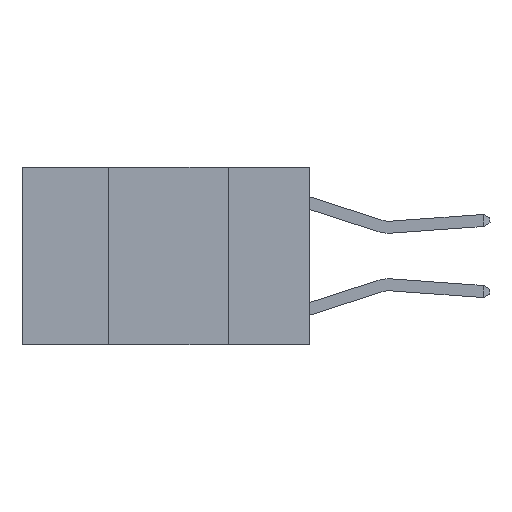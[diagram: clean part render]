
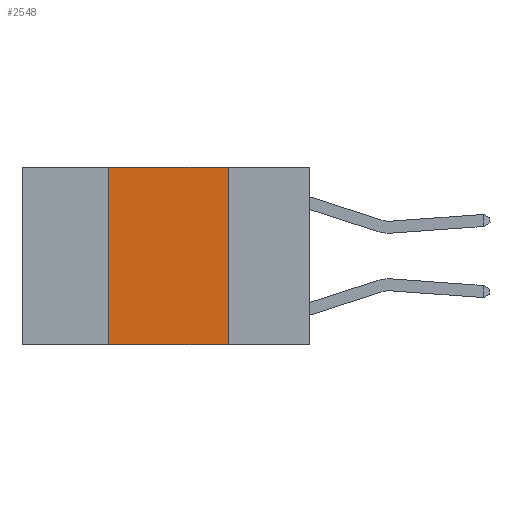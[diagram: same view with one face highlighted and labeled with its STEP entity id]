
A CAD part, left-side view. The second image highlights one B-rep face of the part: STEP entity #2548.
In plain terms, the highlighted planar face has unit normal (-1, 0, 0).
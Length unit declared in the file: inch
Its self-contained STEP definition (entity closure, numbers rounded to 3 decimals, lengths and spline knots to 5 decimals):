
#178 = LINE ( 'NONE', #16218, #3791 ) ;
#269 = EDGE_CURVE ( 'NONE', #16655, #11271, #13785, .T. ) ;
#326 = ORIENTED_EDGE ( 'NONE', *, *, #16401, .F. ) ;
#489 = LINE ( 'NONE', #4417, #16055 ) ;
#1553 = AXIS2_PLACEMENT_3D ( 'NONE', #11176, #2023, #12676 ) ;
#1613 = ORIENTED_EDGE ( 'NONE', *, *, #269, .F. ) ;
#2023 = DIRECTION ( 'NONE',  ( 1., 0., 0. ) ) ;
#2548 = ADVANCED_FACE ( 'NONE', ( #4986 ), #3505, .F. ) ;
#2864 = EDGE_CURVE ( 'NONE', #3091, #16655, #178, .T. ) ;
#2968 = DIRECTION ( 'NONE',  ( 0., -1., 0. ) ) ;
#3091 = VERTEX_POINT ( 'NONE', #4608 ) ;
#3449 = ORIENTED_EDGE ( 'NONE', *, *, #13512, .T. ) ;
#3505 = PLANE ( 'NONE',  #1553 ) ;
#3791 = VECTOR ( 'NONE', #8824, 39.37008 ) ;
#4417 = CARTESIAN_POINT ( 'NONE',  ( 0., 0.6, -0.37 ) ) ;
#4608 = CARTESIAN_POINT ( 'NONE',  ( 0., 0.42, 0. ) ) ;
#4986 = FACE_OUTER_BOUND ( 'NONE', #6889, .T. ) ;
#5318 = LINE ( 'NONE', #16022, #8893 ) ;
#5470 = DIRECTION ( 'NONE',  ( 0., 0., 1. ) ) ;
#6889 = EDGE_LOOP ( 'NONE', ( #1613, #15448, #326, #3449 ) ) ;
#8240 = DIRECTION ( 'NONE',  ( 0., 0., -1. ) ) ;
#8315 = CARTESIAN_POINT ( 'NONE',  ( 0., 0.17, -0.37 ) ) ;
#8824 = DIRECTION ( 'NONE',  ( 0., -1., 0. ) ) ;
#8893 = VECTOR ( 'NONE', #5470, 39.37008 ) ;
#9287 = CARTESIAN_POINT ( 'NONE',  ( 0., 0.17, 0. ) ) ;
#11176 = CARTESIAN_POINT ( 'NONE',  ( 0., 0.6, 0. ) ) ;
#11271 = VERTEX_POINT ( 'NONE', #8315 ) ;
#12676 = DIRECTION ( 'NONE',  ( 0., 0., -1. ) ) ;
#13166 = CARTESIAN_POINT ( 'NONE',  ( 0., 0.42, -0.37 ) ) ;
#13512 = EDGE_CURVE ( 'NONE', #19242, #11271, #489, .T. ) ;
#13785 = LINE ( 'NONE', #9287, #17167 ) ;
#15448 = ORIENTED_EDGE ( 'NONE', *, *, #2864, .F. ) ;
#16022 = CARTESIAN_POINT ( 'NONE',  ( 0., 0.42, 0. ) ) ;
#16055 = VECTOR ( 'NONE', #2968, 39.37008 ) ;
#16218 = CARTESIAN_POINT ( 'NONE',  ( 0., 0.6, 0. ) ) ;
#16401 = EDGE_CURVE ( 'NONE', #19242, #3091, #5318, .T. ) ;
#16487 = CARTESIAN_POINT ( 'NONE',  ( 0., 0.17, 0. ) ) ;
#16655 = VERTEX_POINT ( 'NONE', #16487 ) ;
#17167 = VECTOR ( 'NONE', #8240, 39.37008 ) ;
#19242 = VERTEX_POINT ( 'NONE', #13166 ) ;
